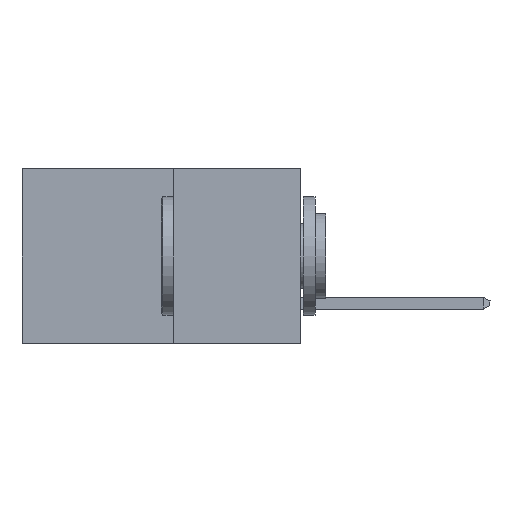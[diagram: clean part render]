
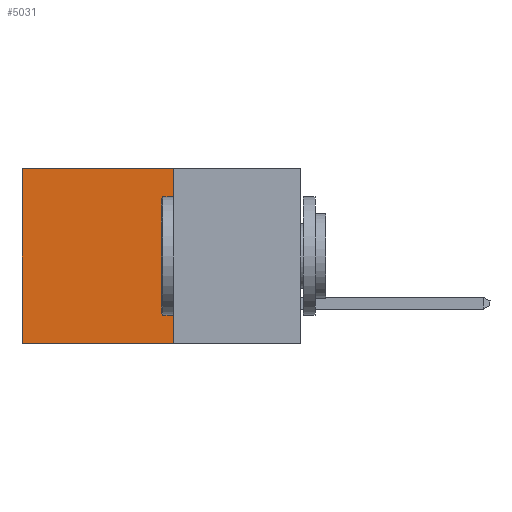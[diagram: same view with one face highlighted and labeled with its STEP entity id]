
A CAD part, left-side view. The second image highlights one B-rep face of the part: STEP entity #5031.
In plain terms, the highlighted planar face has unit normal (-1, 0, 0).
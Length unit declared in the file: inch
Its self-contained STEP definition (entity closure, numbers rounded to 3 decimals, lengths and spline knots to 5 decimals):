
#274 = AXIS2_PLACEMENT_3D ( 'NONE', #12416, #12412, #12397 ) ;
#1621 = EDGE_CURVE ( 'NONE', #9160, #2286, #14267, .T. ) ;
#1674 = LINE ( 'NONE', #13995, #8705 ) ;
#2286 = VERTEX_POINT ( 'NONE', #9859 ) ;
#2290 = CARTESIAN_POINT ( 'NONE',  ( 0.277, 0.59, -0.37 ) ) ;
#2819 = ORIENTED_EDGE ( 'NONE', *, *, #1621, .F. ) ;
#3747 = VECTOR ( 'NONE', #4893, 39.37008 ) ;
#4809 = EDGE_LOOP ( 'NONE', ( #16207, #5714, #2819, #10646 ) ) ;
#4893 = DIRECTION ( 'NONE',  ( 0., 0., -1. ) ) ;
#5031 = ADVANCED_FACE ( 'NONE', ( #17566 ), #12294, .F. ) ;
#5351 = CARTESIAN_POINT ( 'NONE',  ( 0.277, 0.59, 0. ) ) ;
#5714 = ORIENTED_EDGE ( 'NONE', *, *, #9325, .F. ) ;
#5771 = VECTOR ( 'NONE', #13965, 39.37008 ) ;
#8081 = CARTESIAN_POINT ( 'NONE',  ( 0.277, 0.27, 0. ) ) ;
#8705 = VECTOR ( 'NONE', #15414, 39.37008 ) ;
#9069 = VERTEX_POINT ( 'NONE', #2290 ) ;
#9160 = VERTEX_POINT ( 'NONE', #8081 ) ;
#9325 = EDGE_CURVE ( 'NONE', #2286, #9069, #17105, .T. ) ;
#9717 = VERTEX_POINT ( 'NONE', #5351 ) ;
#9859 = CARTESIAN_POINT ( 'NONE',  ( 0.277, 0.27, -0.37 ) ) ;
#10393 = VECTOR ( 'NONE', #13258, 39.37008 ) ;
#10646 = ORIENTED_EDGE ( 'NONE', *, *, #16152, .T. ) ;
#11887 = CARTESIAN_POINT ( 'NONE',  ( 0.277, 0.59, -0.37 ) ) ;
#12294 = PLANE ( 'NONE',  #274 ) ;
#12397 = DIRECTION ( 'NONE',  ( 0., 0., -1. ) ) ;
#12412 = DIRECTION ( 'NONE',  ( 1., 0., 0. ) ) ;
#12416 = CARTESIAN_POINT ( 'NONE',  ( 0.277, 0.27, -0.37 ) ) ;
#13258 = DIRECTION ( 'NONE',  ( 0., 0., -1. ) ) ;
#13965 = DIRECTION ( 'NONE',  ( 0., 1., 0. ) ) ;
#13995 = CARTESIAN_POINT ( 'NONE',  ( 0.277, 0.27, 0. ) ) ;
#14052 = LINE ( 'NONE', #11887, #10393 ) ;
#14267 = LINE ( 'NONE', #16906, #3747 ) ;
#15315 = CARTESIAN_POINT ( 'NONE',  ( 0.277, 0.27, -0.37 ) ) ;
#15414 = DIRECTION ( 'NONE',  ( 0., 1., 0. ) ) ;
#16152 = EDGE_CURVE ( 'NONE', #9160, #9717, #1674, .T. ) ;
#16207 = ORIENTED_EDGE ( 'NONE', *, *, #16470, .T. ) ;
#16470 = EDGE_CURVE ( 'NONE', #9717, #9069, #14052, .T. ) ;
#16906 = CARTESIAN_POINT ( 'NONE',  ( 0.277, 0.27, -0.37 ) ) ;
#17105 = LINE ( 'NONE', #15315, #5771 ) ;
#17566 = FACE_OUTER_BOUND ( 'NONE', #4809, .T. ) ;
